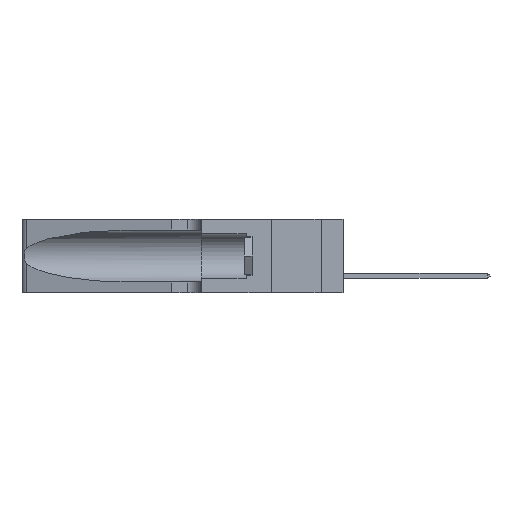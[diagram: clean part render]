
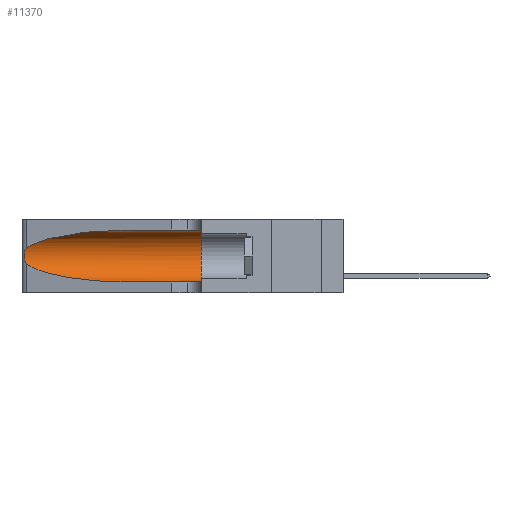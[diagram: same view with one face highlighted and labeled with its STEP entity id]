
A CAD part, left-side view. The second image highlights one B-rep face of the part: STEP entity #11370.
In plain terms, the highlighted cylindrical face has radius 3.308 mm (diameter 6.617 mm), a partial arc.
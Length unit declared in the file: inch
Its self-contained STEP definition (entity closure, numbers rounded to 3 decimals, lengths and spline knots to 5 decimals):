
#180 = EDGE_CURVE ( 'NONE', #20456, #16120, #9839, .T. ) ;
#350 = CARTESIAN_POINT ( 'NONE',  ( 0.1305, 0.72297, 0.31525 ) ) ;
#779 = CARTESIAN_POINT ( 'NONE',  ( 0.25856, 1.23593, 0.16098 ) ) ;
#893 = AXIS2_PLACEMENT_3D ( 'NONE', #22367, #11537, #20911 ) ;
#1140 = EDGE_CURVE ( 'NONE', #20456, #10293, #11663, .T. ) ;
#1241 = EDGE_CURVE ( 'NONE', #10293, #13998, #18991, .T. ) ;
#1245 = DIRECTION ( 'NONE',  ( 0., -1., 0. ) ) ;
#1588 = CYLINDRICAL_SURFACE ( 'NONE', #19247, 0.13025 ) ;
#2254 = CARTESIAN_POINT ( 'NONE',  ( 0.18966, 0.96281, 0.31525 ) ) ;
#2547 = CARTESIAN_POINT ( 'NONE',  ( 0.1305, 1.61858, 0.185 ) ) ;
#3219 = CARTESIAN_POINT ( 'NONE',  ( 0.1305, 0.35, 0.31525 ) ) ;
#3326 = CARTESIAN_POINT ( 'NONE',  ( 0.25487, 1.22718, 0.14631 ) ) ;
#3788 = CARTESIAN_POINT ( 'NONE',  ( 0.25854, 1.2359, 0.20912 ) ) ;
#4004 = CARTESIAN_POINT ( 'NONE',  ( 0.1305, 0.72297, 0.05475 ) ) ;
#4110 = CARTESIAN_POINT ( 'NONE',  ( 0.25487, 1.22718, 0.14631 ) ) ;
#4242 = EDGE_CURVE ( 'NONE', #16120, #18804, #14732, .T. ) ;
#5076 = CARTESIAN_POINT ( 'NONE',  ( 0.1305, 1.61858, 0.05475 ) ) ;
#5970 = ORIENTED_EDGE ( 'NONE', *, *, #1241, .F. ) ;
#6966 = DIRECTION ( 'NONE',  ( 0., -1., 0. ) ) ;
#7394 = CARTESIAN_POINT ( 'NONE',  ( 0.26018, 1.23835, 0.19895 ) ) ;
#7880 = CARTESIAN_POINT ( 'NONE',  ( 0.26075, 1.23896, 0.178 ) ) ;
#8141 = DIRECTION ( 'NONE',  ( 0., 0., -1. ) ) ;
#8294 = CARTESIAN_POINT ( 'NONE',  ( 0.1305, 0.72297, 0.31525 ) ) ;
#9839 =( BOUNDED_CURVE ( )  B_SPLINE_CURVE ( 3, ( #350, #2254, #13125, #11238 ),
 .UNSPECIFIED., .F., .T. ) 
 B_SPLINE_CURVE_WITH_KNOTS ( ( 4, 4 ),
 ( 1.5708, 2.84003 ),
 .UNSPECIFIED. ) 
 CURVE ( )  GEOMETRIC_REPRESENTATION_ITEM ( )  RATIONAL_B_SPLINE_CURVE ( ( 1., 0.87, 0.87, 1. ) ) 
 REPRESENTATION_ITEM ( '' )  );
#10040 = EDGE_CURVE ( 'NONE', #18804, #22337, #12980, .T. ) ;
#10293 = VERTEX_POINT ( 'NONE', #3219 ) ;
#10931 = CARTESIAN_POINT ( 'NONE',  ( 0.25555, 1.22994, 0.2215 ) ) ;
#11065 = CARTESIAN_POINT ( 'NONE',  ( 0.18966, 0.96281, 0.05475 ) ) ;
#11238 = CARTESIAN_POINT ( 'NONE',  ( 0.25487, 1.22718, 0.22369 ) ) ;
#11370 = ADVANCED_FACE ( 'NONE', ( #18235 ), #1588, .F. ) ;
#11537 = DIRECTION ( 'NONE',  ( 0., 1., 0. ) ) ;
#11663 = LINE ( 'NONE', #12203, #14489 ) ;
#12203 = CARTESIAN_POINT ( 'NONE',  ( 0.1305, 1.61858, 0.31525 ) ) ;
#12750 = CARTESIAN_POINT ( 'NONE',  ( 0.25787, 1.23484, 0.2124 ) ) ;
#12980 =( BOUNDED_CURVE ( )  B_SPLINE_CURVE ( 3, ( #20222, #14781, #11065, #4004 ),
 .UNSPECIFIED., .F., .F. ) 
 B_SPLINE_CURVE_WITH_KNOTS ( ( 4, 4 ),
 ( 3.44316, 4.71239 ),
 .UNSPECIFIED. ) 
 CURVE ( )  GEOMETRIC_REPRESENTATION_ITEM ( )  RATIONAL_B_SPLINE_CURVE ( ( 1., 0.87, 0.87, 1. ) ) 
 REPRESENTATION_ITEM ( '' )  );
#13063 = CARTESIAN_POINT ( 'NONE',  ( 0.25555, 1.22993, 0.14849 ) ) ;
#13125 = CARTESIAN_POINT ( 'NONE',  ( 0.2373, 1.15595, 0.28018 ) ) ;
#13998 = VERTEX_POINT ( 'NONE', #18871 ) ;
#14250 = ORIENTED_EDGE ( 'NONE', *, *, #1140, .F. ) ;
#14489 = VECTOR ( 'NONE', #1245, 39.37008 ) ;
#14500 = CARTESIAN_POINT ( 'NONE',  ( 0.25487, 1.22718, 0.22369 ) ) ;
#14732 = B_SPLINE_CURVE_WITH_KNOTS ( 'NONE', 3,
 ( #14500, #10931, #16442, #12750, #3788, #7394, #16850, #7880, #16676, #779, #15211, #17001, #13063, #4110 ),
 .UNSPECIFIED., .F., .F.,
 ( 4, 2, 2, 2, 2, 2, 4 ),
 ( 0., 0.00027, 0.00053, 0.00107, 0.0016, 0.00187, 0.00214 ),
 .UNSPECIFIED. ) ;
#14781 = CARTESIAN_POINT ( 'NONE',  ( 0.2373, 1.15595, 0.08982 ) ) ;
#14813 = ORIENTED_EDGE ( 'NONE', *, *, #4242, .T. ) ;
#15211 = CARTESIAN_POINT ( 'NONE',  ( 0.25789, 1.23486, 0.15765 ) ) ;
#16120 = VERTEX_POINT ( 'NONE', #21110 ) ;
#16442 = CARTESIAN_POINT ( 'NONE',  ( 0.25639, 1.23184, 0.21858 ) ) ;
#16674 = ORIENTED_EDGE ( 'NONE', *, *, #17183, .T. ) ;
#16676 = CARTESIAN_POINT ( 'NONE',  ( 0.26017, 1.23833, 0.17102 ) ) ;
#16850 = CARTESIAN_POINT ( 'NONE',  ( 0.26075, 1.23896, 0.19203 ) ) ;
#16906 = VECTOR ( 'NONE', #6966, 39.37008 ) ;
#17001 = CARTESIAN_POINT ( 'NONE',  ( 0.25639, 1.23186, 0.15144 ) ) ;
#17183 = EDGE_CURVE ( 'NONE', #22337, #13998, #19724, .T. ) ;
#17431 = CARTESIAN_POINT ( 'NONE',  ( 0.1305, 0.72297, 0.05475 ) ) ;
#18235 = FACE_OUTER_BOUND ( 'NONE', #18964, .T. ) ;
#18688 = ORIENTED_EDGE ( 'NONE', *, *, #10040, .T. ) ;
#18804 = VERTEX_POINT ( 'NONE', #3326 ) ;
#18871 = CARTESIAN_POINT ( 'NONE',  ( 0.1305, 0.35, 0.05475 ) ) ;
#18964 = EDGE_LOOP ( 'NONE', ( #22808, #14813, #18688, #16674, #5970, #14250 ) ) ;
#18991 = CIRCLE ( 'NONE', #893, 0.13025 ) ;
#19247 = AXIS2_PLACEMENT_3D ( 'NONE', #2547, #22511, #8141 ) ;
#19724 = LINE ( 'NONE', #5076, #16906 ) ;
#20222 = CARTESIAN_POINT ( 'NONE',  ( 0.25487, 1.22718, 0.14631 ) ) ;
#20456 = VERTEX_POINT ( 'NONE', #8294 ) ;
#20911 = DIRECTION ( 'NONE',  ( 0., 0., 1. ) ) ;
#21110 = CARTESIAN_POINT ( 'NONE',  ( 0.25487, 1.22718, 0.22369 ) ) ;
#22337 = VERTEX_POINT ( 'NONE', #17431 ) ;
#22367 = CARTESIAN_POINT ( 'NONE',  ( 0.1305, 0.35, 0.185 ) ) ;
#22511 = DIRECTION ( 'NONE',  ( 0., -1., 0. ) ) ;
#22808 = ORIENTED_EDGE ( 'NONE', *, *, #180, .T. ) ;
